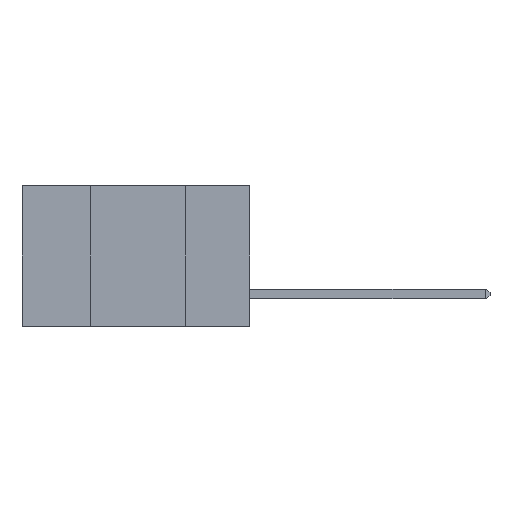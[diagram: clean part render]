
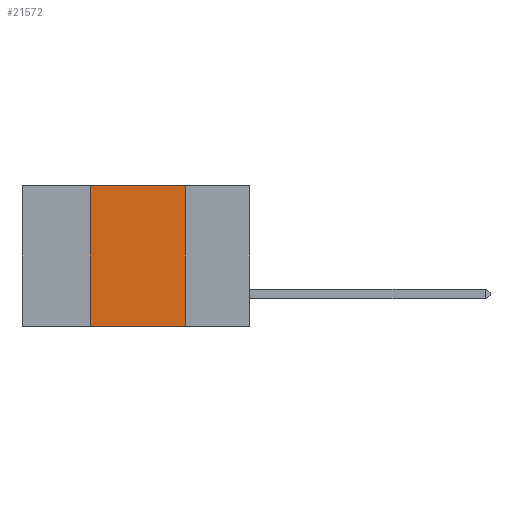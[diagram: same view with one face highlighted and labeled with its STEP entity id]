
A CAD part, left-side view. The second image highlights one B-rep face of the part: STEP entity #21572.
In plain terms, the highlighted planar face has unit normal (-1, 0, 0).
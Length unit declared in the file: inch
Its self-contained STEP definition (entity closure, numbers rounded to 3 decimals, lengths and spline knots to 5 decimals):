
#42 = DIRECTION ( 'NONE',  ( 0., -1., 0. ) ) ;
#1151 = VECTOR ( 'NONE', #19173, 39.37008 ) ;
#1690 = AXIS2_PLACEMENT_3D ( 'NONE', #3873, #9980, #22930 ) ;
#2041 = VERTEX_POINT ( 'NONE', #20312 ) ;
#3232 = LINE ( 'NONE', #15171, #23159 ) ;
#3873 = CARTESIAN_POINT ( 'NONE',  ( 0., 0.6, 0. ) ) ;
#4866 = EDGE_CURVE ( 'NONE', #18186, #8648, #6276, .T. ) ;
#5004 = LINE ( 'NONE', #11640, #19971 ) ;
#5420 = EDGE_CURVE ( 'NONE', #7534, #18186, #13358, .T. ) ;
#6276 = LINE ( 'NONE', #17334, #1151 ) ;
#6778 = CARTESIAN_POINT ( 'NONE',  ( 0., 0.42, 0. ) ) ;
#6896 = ORIENTED_EDGE ( 'NONE', *, *, #17347, .T. ) ;
#7534 = VERTEX_POINT ( 'NONE', #6778 ) ;
#8559 = EDGE_CURVE ( 'NONE', #2041, #7534, #5004, .T. ) ;
#8648 = VERTEX_POINT ( 'NONE', #22940 ) ;
#8922 = ORIENTED_EDGE ( 'NONE', *, *, #4866, .F. ) ;
#9980 = DIRECTION ( 'NONE',  ( 1., 0., 0. ) ) ;
#11640 = CARTESIAN_POINT ( 'NONE',  ( 0., 0.42, 0. ) ) ;
#13358 = LINE ( 'NONE', #13392, #13942 ) ;
#13392 = CARTESIAN_POINT ( 'NONE',  ( 0., 0.6, 0. ) ) ;
#13446 = EDGE_LOOP ( 'NONE', ( #8922, #20593, #17987, #6896 ) ) ;
#13503 = DIRECTION ( 'NONE',  ( 0., 0., 1. ) ) ;
#13942 = VECTOR ( 'NONE', #42, 39.37008 ) ;
#15171 = CARTESIAN_POINT ( 'NONE',  ( 0., 0.6, -0.37 ) ) ;
#16248 = CARTESIAN_POINT ( 'NONE',  ( 0., 0.17, 0. ) ) ;
#16448 = FACE_OUTER_BOUND ( 'NONE', #13446, .T. ) ;
#17038 = DIRECTION ( 'NONE',  ( 0., -1., 0. ) ) ;
#17334 = CARTESIAN_POINT ( 'NONE',  ( 0., 0.17, 0. ) ) ;
#17347 = EDGE_CURVE ( 'NONE', #2041, #8648, #3232, .T. ) ;
#17987 = ORIENTED_EDGE ( 'NONE', *, *, #8559, .F. ) ;
#18186 = VERTEX_POINT ( 'NONE', #16248 ) ;
#19173 = DIRECTION ( 'NONE',  ( 0., 0., -1. ) ) ;
#19971 = VECTOR ( 'NONE', #13503, 39.37008 ) ;
#20312 = CARTESIAN_POINT ( 'NONE',  ( 0., 0.42, -0.37 ) ) ;
#20593 = ORIENTED_EDGE ( 'NONE', *, *, #5420, .F. ) ;
#21107 = PLANE ( 'NONE',  #1690 ) ;
#21572 = ADVANCED_FACE ( 'NONE', ( #16448 ), #21107, .F. ) ;
#22930 = DIRECTION ( 'NONE',  ( 0., 0., -1. ) ) ;
#22940 = CARTESIAN_POINT ( 'NONE',  ( 0., 0.17, -0.37 ) ) ;
#23159 = VECTOR ( 'NONE', #17038, 39.37008 ) ;
